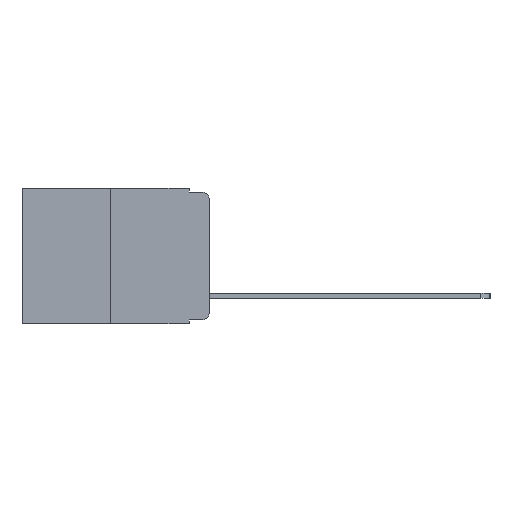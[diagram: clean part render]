
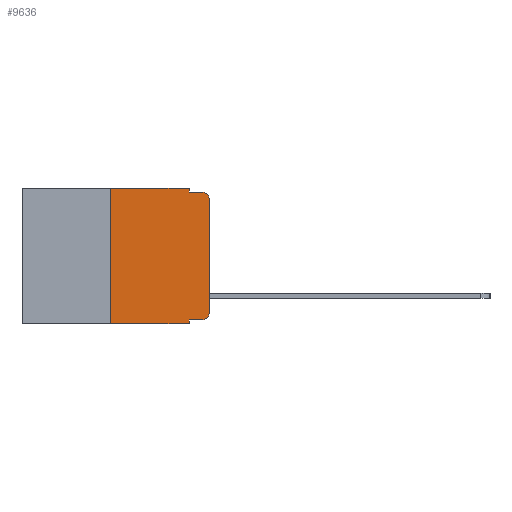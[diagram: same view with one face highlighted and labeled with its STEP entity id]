
A CAD part, left-side view. The second image highlights one B-rep face of the part: STEP entity #9636.
In plain terms, the highlighted planar face has unit normal (-1, 0, 0).
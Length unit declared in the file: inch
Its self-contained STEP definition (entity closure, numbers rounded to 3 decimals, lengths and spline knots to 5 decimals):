
#473 = CARTESIAN_POINT ( 'NONE',  ( 0., 0.02, -0.333 ) ) ;
#719 = DIRECTION ( 'NONE',  ( 0., 0., -1. ) ) ;
#1333 = CARTESIAN_POINT ( 'NONE',  ( 0., 0.02, -0.313 ) ) ;
#1541 = VERTEX_POINT ( 'NONE', #8064 ) ;
#1690 = VECTOR ( 'NONE', #7510, 39.37008 ) ;
#1703 = ORIENTED_EDGE ( 'NONE', *, *, #4977, .T. ) ;
#2154 = DIRECTION ( 'NONE',  ( 0., -1., 0. ) ) ;
#2405 = DIRECTION ( 'NONE',  ( 0., 0., -1. ) ) ;
#2455 = CARTESIAN_POINT ( 'NONE',  ( 0., 0.473, -0.343 ) ) ;
#2680 = CARTESIAN_POINT ( 'NONE',  ( 0., 0.25, -0.343 ) ) ;
#2931 = AXIS2_PLACEMENT_3D ( 'NONE', #1333, #8162, #2405 ) ;
#3262 = EDGE_CURVE ( 'NONE', #4667, #4700, #4558, .T. ) ;
#3303 = EDGE_CURVE ( 'NONE', #7767, #3402, #11529, .T. ) ;
#3402 = VERTEX_POINT ( 'NONE', #9320 ) ;
#3527 = VECTOR ( 'NONE', #8981, 39.37008 ) ;
#3894 = LINE ( 'NONE', #5153, #6146 ) ;
#3960 = VECTOR ( 'NONE', #10122, 39.37008 ) ;
#4233 = CIRCLE ( 'NONE', #10432, 0.02 ) ;
#4335 = CARTESIAN_POINT ( 'NONE',  ( 0., 0.25, 0. ) ) ;
#4351 = ORIENTED_EDGE ( 'NONE', *, *, #12484, .T. ) ;
#4545 = VERTEX_POINT ( 'NONE', #4335 ) ;
#4558 = CIRCLE ( 'NONE', #2931, 0.02 ) ;
#4650 = ORIENTED_EDGE ( 'NONE', *, *, #8119, .F. ) ;
#4651 = PLANE ( 'NONE',  #11326 ) ;
#4667 = VERTEX_POINT ( 'NONE', #473 ) ;
#4700 = VERTEX_POINT ( 'NONE', #8393 ) ;
#4768 = CARTESIAN_POINT ( 'NONE',  ( 0., 0.051, 0. ) ) ;
#4977 = EDGE_CURVE ( 'NONE', #4700, #9206, #6076, .T. ) ;
#5153 = CARTESIAN_POINT ( 'NONE',  ( 0., 0.25, 0. ) ) ;
#5229 = CARTESIAN_POINT ( 'NONE',  ( 0., 0.02, -0.03 ) ) ;
#5615 = DIRECTION ( 'NONE',  ( 0., 0., -1. ) ) ;
#5674 = CARTESIAN_POINT ( 'NONE',  ( 0., 0.473, 0. ) ) ;
#5951 = VERTEX_POINT ( 'NONE', #12168 ) ;
#5961 = LINE ( 'NONE', #8485, #6255 ) ;
#6033 = VECTOR ( 'NONE', #2154, 39.37008 ) ;
#6048 = EDGE_CURVE ( 'NONE', #5951, #8677, #11809, .T. ) ;
#6076 = LINE ( 'NONE', #7003, #3527 ) ;
#6146 = VECTOR ( 'NONE', #10835, 39.37008 ) ;
#6193 = DIRECTION ( 'NONE',  ( 0., 0., -1. ) ) ;
#6255 = VECTOR ( 'NONE', #5615, 39.37008 ) ;
#6330 = LINE ( 'NONE', #11684, #6033 ) ;
#6509 = VERTEX_POINT ( 'NONE', #9483 ) ;
#6625 = DIRECTION ( 'NONE',  ( 0., 0., -1. ) ) ;
#6764 = EDGE_CURVE ( 'NONE', #8677, #6509, #6330, .T. ) ;
#6885 = LINE ( 'NONE', #9427, #1690 ) ;
#6894 = ORIENTED_EDGE ( 'NONE', *, *, #6764, .F. ) ;
#7003 = CARTESIAN_POINT ( 'NONE',  ( 0., 0., 0. ) ) ;
#7189 = ORIENTED_EDGE ( 'NONE', *, *, #3303, .T. ) ;
#7488 = ORIENTED_EDGE ( 'NONE', *, *, #12218, .T. ) ;
#7510 = DIRECTION ( 'NONE',  ( 0., -1., 0. ) ) ;
#7650 = DIRECTION ( 'NONE',  ( 0., -1., 0. ) ) ;
#7705 = CARTESIAN_POINT ( 'NONE',  ( 0., 0., -0.03 ) ) ;
#7767 = VERTEX_POINT ( 'NONE', #2680 ) ;
#7867 = EDGE_LOOP ( 'NONE', ( #1703, #4351, #6894, #9470, #11910, #4650, #7189, #12196, #7488, #10032 ) ) ;
#8060 = FACE_OUTER_BOUND ( 'NONE', #7867, .T. ) ;
#8064 = CARTESIAN_POINT ( 'NONE',  ( 0., 0.051, -0.333 ) ) ;
#8119 = EDGE_CURVE ( 'NONE', #7767, #4545, #3894, .T. ) ;
#8162 = DIRECTION ( 'NONE',  ( -1., 0., 0. ) ) ;
#8393 = CARTESIAN_POINT ( 'NONE',  ( 0., 0., -0.313 ) ) ;
#8485 = CARTESIAN_POINT ( 'NONE',  ( 0., 0.051, 0. ) ) ;
#8571 = CARTESIAN_POINT ( 'NONE',  ( 0., 0.051, -0.333 ) ) ;
#8677 = VERTEX_POINT ( 'NONE', #9955 ) ;
#8737 = VECTOR ( 'NONE', #719, 39.37008 ) ;
#8964 = EDGE_CURVE ( 'NONE', #4545, #5951, #6885, .T. ) ;
#8981 = DIRECTION ( 'NONE',  ( 0., 0., 1. ) ) ;
#9206 = VERTEX_POINT ( 'NONE', #7705 ) ;
#9320 = CARTESIAN_POINT ( 'NONE',  ( 0., 0.051, -0.343 ) ) ;
#9427 = CARTESIAN_POINT ( 'NONE',  ( 0., 0.473, 0. ) ) ;
#9470 = ORIENTED_EDGE ( 'NONE', *, *, #6048, .F. ) ;
#9483 = CARTESIAN_POINT ( 'NONE',  ( 0., 0.02, -0.01 ) ) ;
#9505 = VECTOR ( 'NONE', #7650, 39.37008 ) ;
#9636 = ADVANCED_FACE ( 'NONE', ( #8060 ), #4651, .F. ) ;
#9955 = CARTESIAN_POINT ( 'NONE',  ( 0., 0.051, -0.01 ) ) ;
#10032 = ORIENTED_EDGE ( 'NONE', *, *, #3262, .T. ) ;
#10073 = LINE ( 'NONE', #8571, #9505 ) ;
#10122 = DIRECTION ( 'NONE',  ( 0., -1., 0. ) ) ;
#10202 = EDGE_CURVE ( 'NONE', #1541, #3402, #5961, .T. ) ;
#10432 = AXIS2_PLACEMENT_3D ( 'NONE', #5229, #11843, #6193 ) ;
#10835 = DIRECTION ( 'NONE',  ( 0., 0., 1. ) ) ;
#11326 = AXIS2_PLACEMENT_3D ( 'NONE', #5674, #12260, #6625 ) ;
#11529 = LINE ( 'NONE', #2455, #3960 ) ;
#11684 = CARTESIAN_POINT ( 'NONE',  ( 0., 0.051, -0.01 ) ) ;
#11809 = LINE ( 'NONE', #4768, #8737 ) ;
#11843 = DIRECTION ( 'NONE',  ( -1., 0., 0. ) ) ;
#11910 = ORIENTED_EDGE ( 'NONE', *, *, #8964, .F. ) ;
#12168 = CARTESIAN_POINT ( 'NONE',  ( 0., 0.051, 0. ) ) ;
#12196 = ORIENTED_EDGE ( 'NONE', *, *, #10202, .F. ) ;
#12218 = EDGE_CURVE ( 'NONE', #1541, #4667, #10073, .T. ) ;
#12260 = DIRECTION ( 'NONE',  ( 1., 0., 0. ) ) ;
#12484 = EDGE_CURVE ( 'NONE', #9206, #6509, #4233, .T. ) ;
